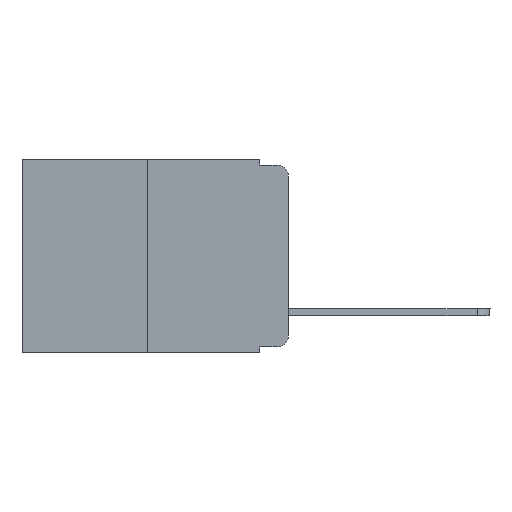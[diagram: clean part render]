
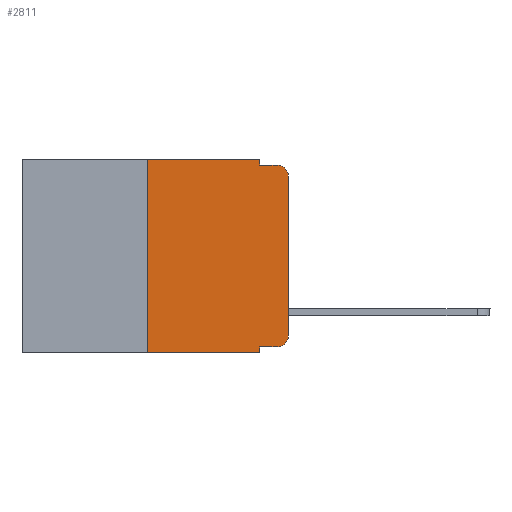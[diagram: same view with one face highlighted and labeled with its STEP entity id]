
A CAD part, left-side view. The second image highlights one B-rep face of the part: STEP entity #2811.
In plain terms, the highlighted planar face has unit normal (-1, 0, 0).
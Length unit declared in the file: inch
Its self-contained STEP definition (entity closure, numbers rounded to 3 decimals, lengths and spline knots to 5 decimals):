
#341 = DIRECTION ( 'NONE',  ( 1., 0., 0. ) ) ;
#406 = VERTEX_POINT ( 'NONE', #1227 ) ;
#433 = VECTOR ( 'NONE', #9551, 39.37008 ) ;
#449 = CARTESIAN_POINT ( 'NONE',  ( 0., 0.02, -0.313 ) ) ;
#1227 = CARTESIAN_POINT ( 'NONE',  ( 0., 0.051, -0.343 ) ) ;
#1295 = EDGE_CURVE ( 'NONE', #14942, #406, #14050, .T. ) ;
#1965 = CARTESIAN_POINT ( 'NONE',  ( 0., 0.051, -0.01 ) ) ;
#1977 = ORIENTED_EDGE ( 'NONE', *, *, #8144, .T. ) ;
#2057 = CIRCLE ( 'NONE', #5661, 0.02 ) ;
#2065 = CARTESIAN_POINT ( 'NONE',  ( 0., 0., -0.03 ) ) ;
#2069 = EDGE_CURVE ( 'NONE', #14942, #5971, #16614, .T. ) ;
#2122 = DIRECTION ( 'NONE',  ( 0., 0., -1. ) ) ;
#2176 = CARTESIAN_POINT ( 'NONE',  ( 0., 0.051, 0. ) ) ;
#2196 = LINE ( 'NONE', #6642, #10215 ) ;
#2227 = EDGE_CURVE ( 'NONE', #18645, #6019, #2196, .T. ) ;
#2811 = ADVANCED_FACE ( 'NONE', ( #7626 ), #10829, .F. ) ;
#2822 = CARTESIAN_POINT ( 'NONE',  ( 0., 0.473, 0. ) ) ;
#3314 = CARTESIAN_POINT ( 'NONE',  ( 0., 0.02, -0.03 ) ) ;
#3666 = DIRECTION ( 'NONE',  ( 0., 0., 1. ) ) ;
#4632 = ORIENTED_EDGE ( 'NONE', *, *, #8106, .F. ) ;
#4741 = ORIENTED_EDGE ( 'NONE', *, *, #11897, .F. ) ;
#4779 = CARTESIAN_POINT ( 'NONE',  ( 0., 0.02, -0.333 ) ) ;
#4995 = ORIENTED_EDGE ( 'NONE', *, *, #2069, .T. ) ;
#5202 = CARTESIAN_POINT ( 'NONE',  ( 0., 0.25, -0.343 ) ) ;
#5584 = VERTEX_POINT ( 'NONE', #2065 ) ;
#5661 = AXIS2_PLACEMENT_3D ( 'NONE', #3314, #15264, #7684 ) ;
#5772 = DIRECTION ( 'NONE',  ( 0., 0., 1. ) ) ;
#5971 = VERTEX_POINT ( 'NONE', #4779 ) ;
#6019 = VERTEX_POINT ( 'NONE', #7322 ) ;
#6096 = VECTOR ( 'NONE', #18330, 39.37008 ) ;
#6642 = CARTESIAN_POINT ( 'NONE',  ( 0., 0.25, 0. ) ) ;
#7017 = AXIS2_PLACEMENT_3D ( 'NONE', #449, #17076, #15633 ) ;
#7291 = CARTESIAN_POINT ( 'NONE',  ( 0., 0.02, -0.01 ) ) ;
#7322 = CARTESIAN_POINT ( 'NONE',  ( 0., 0.25, 0. ) ) ;
#7626 = FACE_OUTER_BOUND ( 'NONE', #15553, .T. ) ;
#7684 = DIRECTION ( 'NONE',  ( 0., 0., -1. ) ) ;
#8106 = EDGE_CURVE ( 'NONE', #16172, #19492, #17658, .T. ) ;
#8144 = EDGE_CURVE ( 'NONE', #18645, #406, #8936, .T. ) ;
#8322 = ORIENTED_EDGE ( 'NONE', *, *, #17366, .T. ) ;
#8715 = AXIS2_PLACEMENT_3D ( 'NONE', #9385, #341, #2122 ) ;
#8928 = ORIENTED_EDGE ( 'NONE', *, *, #1295, .F. ) ;
#8936 = LINE ( 'NONE', #17004, #433 ) ;
#9127 = CARTESIAN_POINT ( 'NONE',  ( 0., 0.051, 0. ) ) ;
#9205 = DIRECTION ( 'NONE',  ( 0., -1., 0. ) ) ;
#9229 = EDGE_CURVE ( 'NONE', #5584, #19492, #2057, .T. ) ;
#9385 = CARTESIAN_POINT ( 'NONE',  ( 0., 0.473, 0. ) ) ;
#9518 = CARTESIAN_POINT ( 'NONE',  ( 0., 0.051, -0.333 ) ) ;
#9551 = DIRECTION ( 'NONE',  ( 0., -1., 0. ) ) ;
#9923 = EDGE_CURVE ( 'NONE', #11745, #16172, #14720, .T. ) ;
#10215 = VECTOR ( 'NONE', #3666, 39.37008 ) ;
#10228 = ORIENTED_EDGE ( 'NONE', *, *, #9923, .F. ) ;
#10321 = ORIENTED_EDGE ( 'NONE', *, *, #19418, .T. ) ;
#10567 = CIRCLE ( 'NONE', #7017, 0.02 ) ;
#10717 = CARTESIAN_POINT ( 'NONE',  ( 0., 0.051, -0.333 ) ) ;
#10829 = PLANE ( 'NONE',  #8715 ) ;
#11104 = LINE ( 'NONE', #13422, #19131 ) ;
#11123 = VECTOR ( 'NONE', #17870, 39.37008 ) ;
#11371 = CARTESIAN_POINT ( 'NONE',  ( 0., 0.051, -0.01 ) ) ;
#11745 = VERTEX_POINT ( 'NONE', #9127 ) ;
#11897 = EDGE_CURVE ( 'NONE', #6019, #11745, #15147, .T. ) ;
#13079 = VECTOR ( 'NONE', #18859, 39.37008 ) ;
#13129 = CARTESIAN_POINT ( 'NONE',  ( 0., 0., -0.313 ) ) ;
#13416 = ORIENTED_EDGE ( 'NONE', *, *, #2227, .F. ) ;
#13422 = CARTESIAN_POINT ( 'NONE',  ( 0., 0., 0. ) ) ;
#13789 = VECTOR ( 'NONE', #9205, 39.37008 ) ;
#14050 = LINE ( 'NONE', #18549, #19458 ) ;
#14720 = LINE ( 'NONE', #2176, #13079 ) ;
#14942 = VERTEX_POINT ( 'NONE', #9518 ) ;
#15105 = VERTEX_POINT ( 'NONE', #13129 ) ;
#15147 = LINE ( 'NONE', #2822, #11123 ) ;
#15264 = DIRECTION ( 'NONE',  ( -1., 0., 0. ) ) ;
#15304 = ORIENTED_EDGE ( 'NONE', *, *, #9229, .T. ) ;
#15553 = EDGE_LOOP ( 'NONE', ( #10321, #15304, #4632, #10228, #4741, #13416, #1977, #8928, #4995, #8322 ) ) ;
#15633 = DIRECTION ( 'NONE',  ( 0., 0., -1. ) ) ;
#16172 = VERTEX_POINT ( 'NONE', #11371 ) ;
#16614 = LINE ( 'NONE', #10717, #13789 ) ;
#16890 = DIRECTION ( 'NONE',  ( 0., 0., -1. ) ) ;
#17004 = CARTESIAN_POINT ( 'NONE',  ( 0., 0.473, -0.343 ) ) ;
#17076 = DIRECTION ( 'NONE',  ( -1., 0., 0. ) ) ;
#17366 = EDGE_CURVE ( 'NONE', #5971, #15105, #10567, .T. ) ;
#17658 = LINE ( 'NONE', #1965, #6096 ) ;
#17870 = DIRECTION ( 'NONE',  ( 0., -1., 0. ) ) ;
#18330 = DIRECTION ( 'NONE',  ( 0., -1., 0. ) ) ;
#18549 = CARTESIAN_POINT ( 'NONE',  ( 0., 0.051, 0. ) ) ;
#18645 = VERTEX_POINT ( 'NONE', #5202 ) ;
#18859 = DIRECTION ( 'NONE',  ( 0., 0., -1. ) ) ;
#19131 = VECTOR ( 'NONE', #5772, 39.37008 ) ;
#19418 = EDGE_CURVE ( 'NONE', #15105, #5584, #11104, .T. ) ;
#19458 = VECTOR ( 'NONE', #16890, 39.37008 ) ;
#19492 = VERTEX_POINT ( 'NONE', #7291 ) ;
